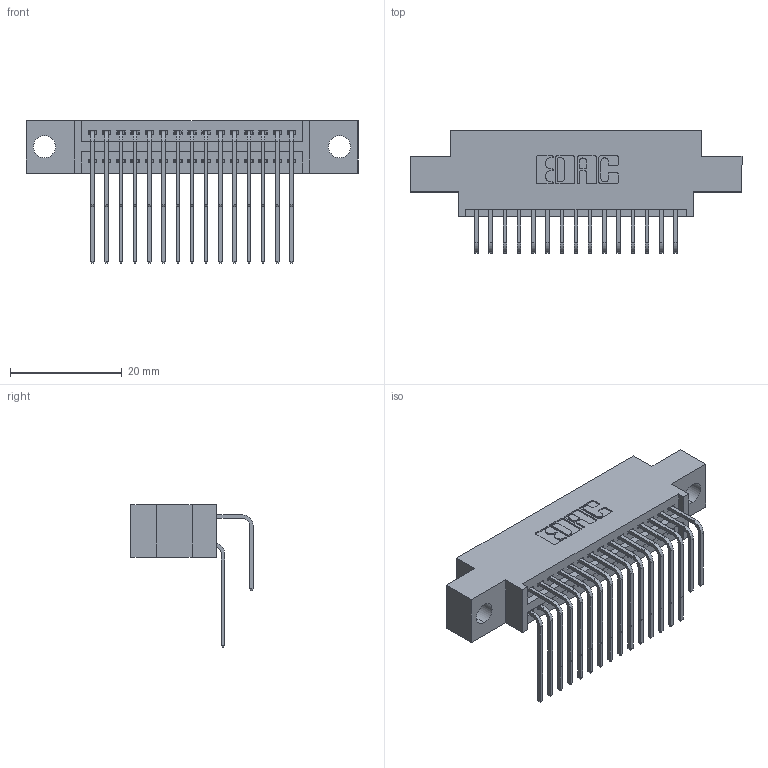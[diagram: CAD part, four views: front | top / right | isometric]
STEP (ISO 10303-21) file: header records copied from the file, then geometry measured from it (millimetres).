
FILE_DESCRIPTION (( 'STEP AP203' ), '1' );
FILE_NAME ('395-030-558-804.STEP', '2021-06-16T20:16:47', ( '' ), ( '' ), 'SwSTEP 2.0', 'SolidWorks 2020', '' );
FILE_SCHEMA (( 'CONFIG_CONTROL_DESIGN' ));
Length unit declared in the file: inch
Products named in the file (4): 345-292-001_558 Tail - 2; 345-292-001_558 559 Tail - 1; 345 Part_0.170 Offset - 0.156 Dia-TI; 395-030-558-804
Assembly tree (31 placements, depth 2):
  395-030-558-804
    345 Part_0.170 Offset - 0.156 Dia-TI
    345-292-001_558 559 Tail - 1  x15
    345-292-001_558 Tail - 2  x15
Bounding box: 59.31 x 21.83 x 25.53 mm (x, y, z)
Volume: 5464.4 mm3; surface area: 8363.3 mm2
Topology: 31 solids, 31 shells, 1704 faces, 5039 edges, 3318 vertices
Faces by surface type: plane 1148, cylinder 556
Entity records: 17607 total; most frequent: CARTESIAN_POINT 3029, ORIENTED_EDGE 2910, DIRECTION 2675, EDGE_CURVE 1455, LINE 1223, VECTOR 1223, VERTEX_POINT 966, AXIS2_PLACEMENT_3D 726
